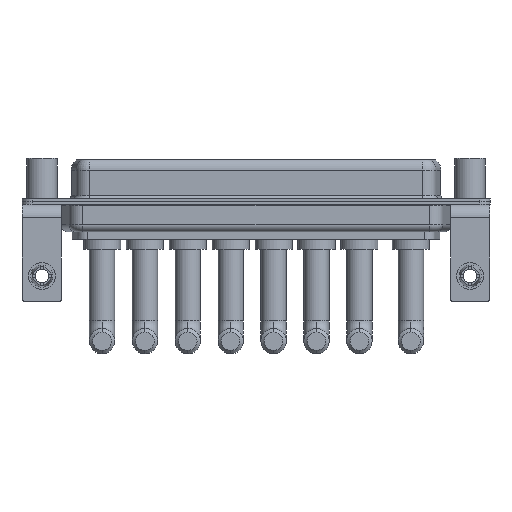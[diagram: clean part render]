
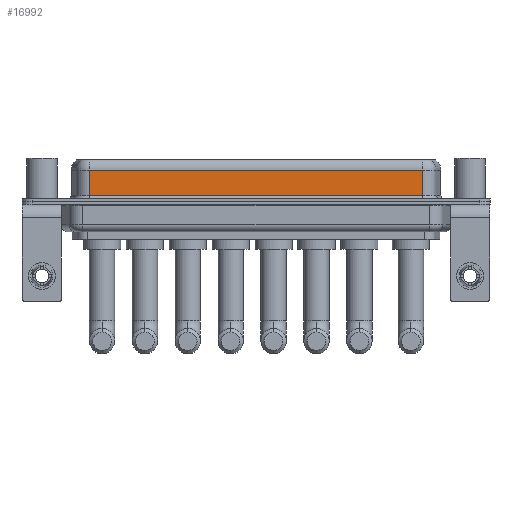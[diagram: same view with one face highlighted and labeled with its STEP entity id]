
A CAD part, front view. The second image highlights one B-rep face of the part: STEP entity #16992.
In plain terms, the highlighted planar face has unit normal (0, -1, 0).
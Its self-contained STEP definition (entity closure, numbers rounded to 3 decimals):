
#2 = LINE ( 'NONE', #10782, #14742 ) ;
#37 = VERTEX_POINT ( 'NONE', #3951 ) ;
#419 = PLANE ( 'NONE',  #2489 ) ;
#602 = ORIENTED_EDGE ( 'NONE', *, *, #6470, .T. ) ;
#1408 = ORIENTED_EDGE ( 'NONE', *, *, #7635, .T. ) ;
#1737 = DIRECTION ( 'NONE',  ( 0., 0., 1. ) ) ;
#1931 = CARTESIAN_POINT ( 'NONE',  ( 56.462, -3.95, 4.65 ) ) ;
#2306 = DIRECTION ( 'NONE',  ( 1., 0., 0. ) ) ;
#2489 = AXIS2_PLACEMENT_3D ( 'NONE', #11178, #9459, #1737 ) ;
#3315 = CARTESIAN_POINT ( 'NONE',  ( 56.462, -3.95, 4.65 ) ) ;
#3951 = CARTESIAN_POINT ( 'NONE',  ( 7.038, -3.95, 4.65 ) ) ;
#4044 = CARTESIAN_POINT ( 'NONE',  ( 56.462, -3.95, 0.9 ) ) ;
#4580 = ORIENTED_EDGE ( 'NONE', *, *, #16900, .T. ) ;
#4585 = ORIENTED_EDGE ( 'NONE', *, *, #11529, .F. ) ;
#5800 = FACE_OUTER_BOUND ( 'NONE', #12646, .T. ) ;
#6470 = EDGE_CURVE ( 'NONE', #37, #6732, #2, .T. ) ;
#6732 = VERTEX_POINT ( 'NONE', #11547 ) ;
#6856 = DIRECTION ( 'NONE',  ( 0., 0., -1. ) ) ;
#7063 = DIRECTION ( 'NONE',  ( -1., 0., 0. ) ) ;
#7635 = EDGE_CURVE ( 'NONE', #13868, #37, #13931, .T. ) ;
#7941 = CARTESIAN_POINT ( 'NONE',  ( 56.462, -3.95, 6.4 ) ) ;
#9459 = DIRECTION ( 'NONE',  ( 0., 1., 0. ) ) ;
#10782 = CARTESIAN_POINT ( 'NONE',  ( 7.038, -3.95, 6.4 ) ) ;
#11178 = CARTESIAN_POINT ( 'NONE',  ( 56.462, -3.95, 6.4 ) ) ;
#11439 = VERTEX_POINT ( 'NONE', #4044 ) ;
#11529 = EDGE_CURVE ( 'NONE', #13868, #11439, #15808, .T. ) ;
#11547 = CARTESIAN_POINT ( 'NONE',  ( 7.038, -3.95, 0.9 ) ) ;
#12646 = EDGE_LOOP ( 'NONE', ( #4585, #1408, #602, #4580 ) ) ;
#13130 = CARTESIAN_POINT ( 'NONE',  ( 56.462, -3.95, 0.9 ) ) ;
#13473 = VECTOR ( 'NONE', #2306, 1000. ) ;
#13570 = DIRECTION ( 'NONE',  ( 0., 0., -1. ) ) ;
#13868 = VERTEX_POINT ( 'NONE', #3315 ) ;
#13931 = LINE ( 'NONE', #1931, #14791 ) ;
#14742 = VECTOR ( 'NONE', #13570, 1000. ) ;
#14791 = VECTOR ( 'NONE', #7063, 1000. ) ;
#15788 = LINE ( 'NONE', #13130, #13473 ) ;
#15808 = LINE ( 'NONE', #7941, #17171 ) ;
#16900 = EDGE_CURVE ( 'NONE', #6732, #11439, #15788, .T. ) ;
#16992 = ADVANCED_FACE ( 'NONE', ( #5800 ), #419, .F. ) ;
#17171 = VECTOR ( 'NONE', #6856, 1000. ) ;
